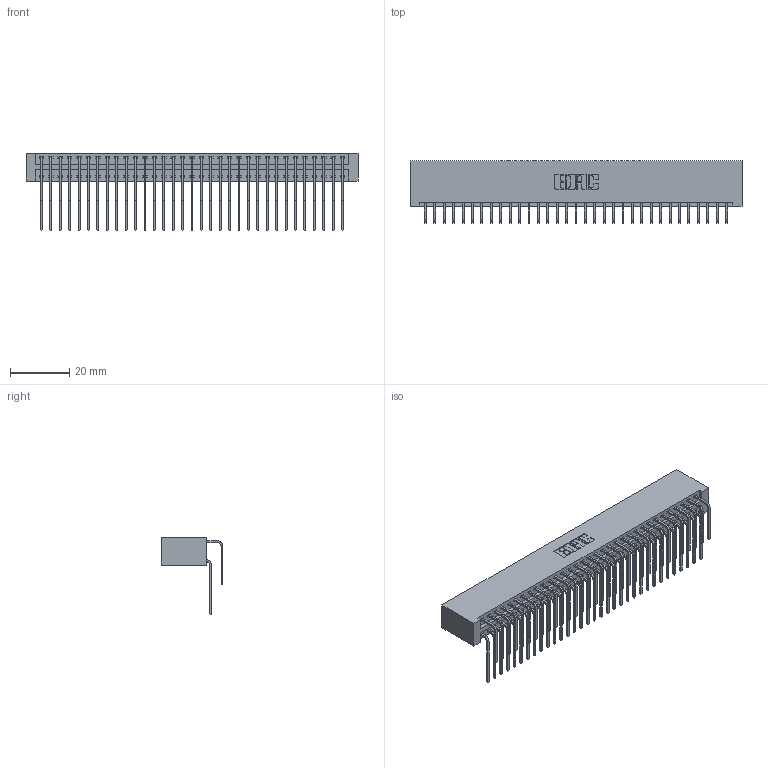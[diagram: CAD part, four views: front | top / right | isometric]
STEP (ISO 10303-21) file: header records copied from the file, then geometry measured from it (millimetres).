
FILE_DESCRIPTION (( 'STEP AP203' ), '1' );
FILE_NAME ('346-066-559-201.STEP', '2022-05-24T18:03:21', ( '' ), ( '' ), 'SwSTEP 2.0', 'SolidWorks 2020', '' );
FILE_SCHEMA (( 'CONFIG_CONTROL_DESIGN' ));
Length unit declared in the file: inch
Products named in the file (4): 346 Part_No Mounting Lugs; 346-066-559-201; 345-292-001_558 559 Tail - 1; 345-292-001_559 Tail - 2
Assembly tree (67 placements, depth 2):
  346-066-559-201
    346 Part_No Mounting Lugs
    345-292-001_558 559 Tail - 1  x33
    345-292-001_559 Tail - 2  x33
Bounding box: 112.01 x 20.89 x 26.16 mm (x, y, z)
Volume: 11806.9 mm3; surface area: 18077.6 mm2
Topology: 67 solids, 67 shells, 3678 faces, 10931 edges, 7198 vertices
Faces by surface type: plane 2514, cylinder 1164
Entity records: 24255 total; most frequent: CARTESIAN_POINT 4059, ORIENTED_EDGE 3942, DIRECTION 3595, EDGE_CURVE 1971, VECTOR 1675, LINE 1675, VERTEX_POINT 1310, AXIS2_PLACEMENT_3D 960
